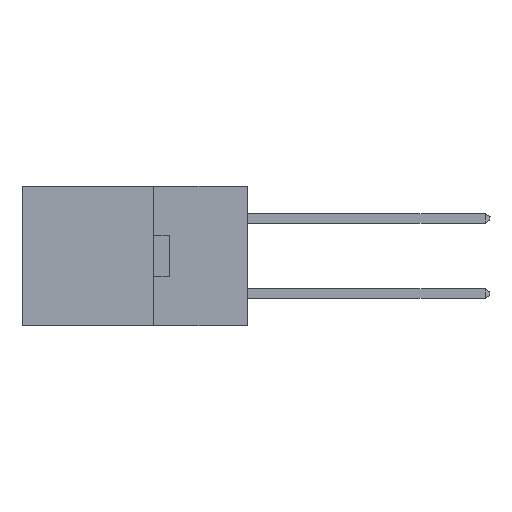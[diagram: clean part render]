
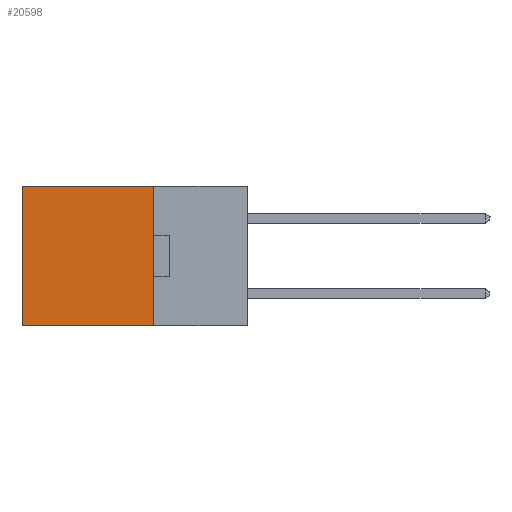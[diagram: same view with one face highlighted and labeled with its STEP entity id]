
A CAD part, left-side view. The second image highlights one B-rep face of the part: STEP entity #20598.
In plain terms, the highlighted planar face has unit normal (-1, 0, 0).
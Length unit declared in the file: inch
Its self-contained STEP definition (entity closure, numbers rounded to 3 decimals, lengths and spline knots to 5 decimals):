
#1489 = CARTESIAN_POINT ( 'NONE',  ( 0.2615, 0.25, 0. ) ) ;
#1898 = VECTOR ( 'NONE', #11954, 39.37008 ) ;
#3105 = CARTESIAN_POINT ( 'NONE',  ( 0.2615, 0.25, -0.37 ) ) ;
#3197 = CARTESIAN_POINT ( 'NONE',  ( 0.2615, 0.25, -0.37 ) ) ;
#3228 = DIRECTION ( 'NONE',  ( 0., 0., -1. ) ) ;
#3475 = LINE ( 'NONE', #3197, #5883 ) ;
#4684 = ORIENTED_EDGE ( 'NONE', *, *, #22915, .T. ) ;
#5164 = EDGE_CURVE ( 'NONE', #21537, #5340, #14071, .T. ) ;
#5340 = VERTEX_POINT ( 'NONE', #15067 ) ;
#5596 = CARTESIAN_POINT ( 'NONE',  ( 0.2615, 0.25, -0.37 ) ) ;
#5699 = AXIS2_PLACEMENT_3D ( 'NONE', #22800, #11397, #3228 ) ;
#5777 = DIRECTION ( 'NONE',  ( 0., 1., 0. ) ) ;
#5883 = VECTOR ( 'NONE', #18506, 39.37008 ) ;
#7513 = FACE_OUTER_BOUND ( 'NONE', #8248, .T. ) ;
#7668 = CARTESIAN_POINT ( 'NONE',  ( 0.2615, 0.25, 0. ) ) ;
#7802 = VERTEX_POINT ( 'NONE', #26301 ) ;
#8248 = EDGE_LOOP ( 'NONE', ( #4684, #27959, #14005, #19102 ) ) ;
#11397 = DIRECTION ( 'NONE',  ( 1., 0., 0. ) ) ;
#11639 = VECTOR ( 'NONE', #19255, 39.37008 ) ;
#11954 = DIRECTION ( 'NONE',  ( 0., 0., -1. ) ) ;
#12375 = CARTESIAN_POINT ( 'NONE',  ( 0.2615, 0.6, -0.37 ) ) ;
#14005 = ORIENTED_EDGE ( 'NONE', *, *, #16044, .F. ) ;
#14071 = LINE ( 'NONE', #1489, #18056 ) ;
#15067 = CARTESIAN_POINT ( 'NONE',  ( 0.2615, 0.6, 0. ) ) ;
#16044 = EDGE_CURVE ( 'NONE', #21537, #23919, #27416, .T. ) ;
#16249 = PLANE ( 'NONE',  #5699 ) ;
#18056 = VECTOR ( 'NONE', #5777, 39.37008 ) ;
#18506 = DIRECTION ( 'NONE',  ( 0., 1., 0. ) ) ;
#19102 = ORIENTED_EDGE ( 'NONE', *, *, #5164, .T. ) ;
#19255 = DIRECTION ( 'NONE',  ( 0., 0., -1. ) ) ;
#20598 = ADVANCED_FACE ( 'NONE', ( #7513 ), #16249, .F. ) ;
#21101 = LINE ( 'NONE', #12375, #11639 ) ;
#21537 = VERTEX_POINT ( 'NONE', #7668 ) ;
#22800 = CARTESIAN_POINT ( 'NONE',  ( 0.2615, 0.25, -0.37 ) ) ;
#22915 = EDGE_CURVE ( 'NONE', #5340, #7802, #21101, .T. ) ;
#23919 = VERTEX_POINT ( 'NONE', #5596 ) ;
#26301 = CARTESIAN_POINT ( 'NONE',  ( 0.2615, 0.6, -0.37 ) ) ;
#27416 = LINE ( 'NONE', #3105, #1898 ) ;
#27576 = EDGE_CURVE ( 'NONE', #23919, #7802, #3475, .T. ) ;
#27959 = ORIENTED_EDGE ( 'NONE', *, *, #27576, .F. ) ;
